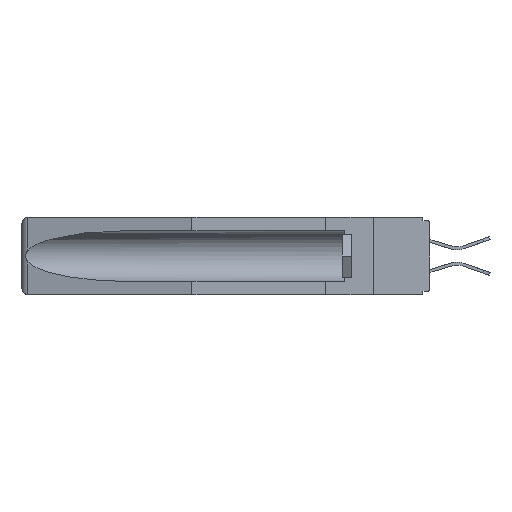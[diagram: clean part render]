
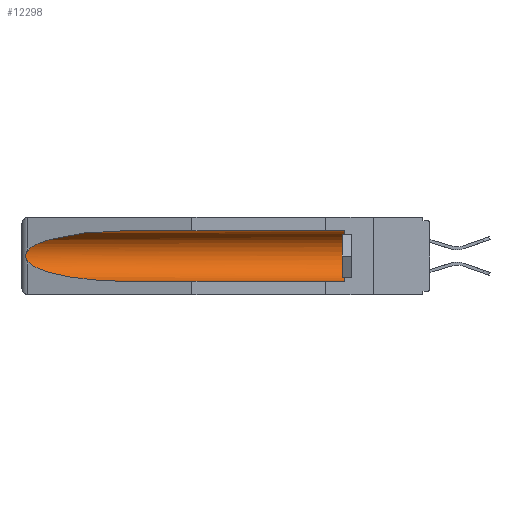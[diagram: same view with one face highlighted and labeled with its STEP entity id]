
A CAD part, left-side view. The second image highlights one B-rep face of the part: STEP entity #12298.
In plain terms, the highlighted cylindrical face has radius 2.857 mm (diameter 5.715 mm), a partial arc.
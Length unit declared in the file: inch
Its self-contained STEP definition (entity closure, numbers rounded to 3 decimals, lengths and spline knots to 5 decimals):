
#168 = CARTESIAN_POINT ( 'NONE',  ( 0.26597, 1.5296, -0.19026 ) ) ;
#405 = CARTESIAN_POINT ( 'NONE',  ( 0.2673, 1.53269, -0.17917 ) ) ;
#1002 = CARTESIAN_POINT ( 'NONE',  ( 0.155, 1.07973, -0.059 ) ) ;
#1911 = ORIENTED_EDGE ( 'NONE', *, *, #16237, .T. ) ;
#3357 = B_SPLINE_CURVE_WITH_KNOTS ( 'NONE', 3,
 ( #9916, #6105, #11764, #21163, #11851, #11530, #405, #13508, #168, #13671 ),
 .UNSPECIFIED., .F., .F.,
 ( 4, 2, 2, 2, 4 ),
 ( 0., 0.00029, 0.00058, 0.00087, 0.00117 ),
 .UNSPECIFIED. ) ;
#3642 = DIRECTION ( 'NONE',  ( 0., 0., 1. ) ) ;
#3734 = ORIENTED_EDGE ( 'NONE', *, *, #9068, .F. ) ;
#3971 = VECTOR ( 'NONE', #6389, 39.37008 ) ;
#4084 = AXIS2_PLACEMENT_3D ( 'NONE', #11189, #5364, #3642 ) ;
#4534 = CARTESIAN_POINT ( 'NONE',  ( 0.26537, 1.52718, -0.19328 ) ) ;
#5364 = DIRECTION ( 'NONE',  ( 0., 1., 0. ) ) ;
#5437 = DIRECTION ( 'NONE',  ( 0., 0., 1. ) ) ;
#5615 = CARTESIAN_POINT ( 'NONE',  ( 0.155, 0.126, -0.1715 ) ) ;
#6105 = CARTESIAN_POINT ( 'NONE',  ( 0.26597, 1.52961, -0.15275 ) ) ;
#6367 = EDGE_CURVE ( 'NONE', #6925, #9127, #13152, .T. ) ;
#6389 = DIRECTION ( 'NONE',  ( 0., 1., 0. ) ) ;
#6392 = CARTESIAN_POINT ( 'NONE',  ( 0.21114, 1.30732, -0.284 ) ) ;
#6740 = CYLINDRICAL_SURFACE ( 'NONE', #4084, 0.1125 ) ;
#6925 = VERTEX_POINT ( 'NONE', #13008 ) ;
#7333 = CARTESIAN_POINT ( 'NONE',  ( 0.155, -0.30754, -0.059 ) ) ;
#7741 = AXIS2_PLACEMENT_3D ( 'NONE', #5615, #9327, #5437 ) ;
#7800 = EDGE_CURVE ( 'NONE', #15560, #8006, #3357, .T. ) ;
#8006 = VERTEX_POINT ( 'NONE', #4534 ) ;
#8817 = FACE_OUTER_BOUND ( 'NONE', #18758, .T. ) ;
#9068 = EDGE_CURVE ( 'NONE', #17159, #22945, #17470, .T. ) ;
#9127 = VERTEX_POINT ( 'NONE', #13277 ) ;
#9134 = ORIENTED_EDGE ( 'NONE', *, *, #6367, .T. ) ;
#9327 = DIRECTION ( 'NONE',  ( 0., -1., 0. ) ) ;
#9916 = CARTESIAN_POINT ( 'NONE',  ( 0.26537, 1.52718, -0.14972 ) ) ;
#10956 = DIRECTION ( 'NONE',  ( 0., 1., 0. ) ) ;
#11189 = CARTESIAN_POINT ( 'NONE',  ( 0.155, -0.30754, -0.1715 ) ) ;
#11530 = CARTESIAN_POINT ( 'NONE',  ( 0.2675, 1.53308, -0.17534 ) ) ;
#11764 = CARTESIAN_POINT ( 'NONE',  ( 0.26654, 1.53092, -0.15636 ) ) ;
#11851 = CARTESIAN_POINT ( 'NONE',  ( 0.2675, 1.53308, -0.16763 ) ) ;
#12298 = ADVANCED_FACE ( 'NONE', ( #8817 ), #6740, .F. ) ;
#13008 = CARTESIAN_POINT ( 'NONE',  ( 0.155, 0.126, -0.059 ) ) ;
#13152 = LINE ( 'NONE', #7333, #3971 ) ;
#13276 = ORIENTED_EDGE ( 'NONE', *, *, #7800, .T. ) ;
#13277 = CARTESIAN_POINT ( 'NONE',  ( 0.155, 1.07973, -0.059 ) ) ;
#13508 = CARTESIAN_POINT ( 'NONE',  ( 0.26655, 1.53094, -0.18657 ) ) ;
#13671 = CARTESIAN_POINT ( 'NONE',  ( 0.26537, 1.52718, -0.19328 ) ) ;
#14154 = EDGE_CURVE ( 'NONE', #9127, #15560, #22742, .T. ) ;
#14417 = CARTESIAN_POINT ( 'NONE',  ( 0.26537, 1.52718, -0.14972 ) ) ;
#14963 = CARTESIAN_POINT ( 'NONE',  ( 0.155, 0.126, -0.284 ) ) ;
#15560 = VERTEX_POINT ( 'NONE', #19861 ) ;
#16156 = CARTESIAN_POINT ( 'NONE',  ( 0.21114, 1.30732, -0.059 ) ) ;
#16237 = EDGE_CURVE ( 'NONE', #8006, #22945, #20940, .T. ) ;
#16647 = CARTESIAN_POINT ( 'NONE',  ( 0.155, -0.30754, -0.284 ) ) ;
#17159 = VERTEX_POINT ( 'NONE', #14963 ) ;
#17470 = LINE ( 'NONE', #16647, #17757 ) ;
#17757 = VECTOR ( 'NONE', #10956, 39.37008 ) ;
#18758 = EDGE_LOOP ( 'NONE', ( #23202, #13276, #1911, #3734, #22509, #9134 ) ) ;
#19003 = CARTESIAN_POINT ( 'NONE',  ( 0.155, 1.07973, -0.284 ) ) ;
#19468 = CARTESIAN_POINT ( 'NONE',  ( 0.25451, 1.48313, -0.24835 ) ) ;
#19539 = CARTESIAN_POINT ( 'NONE',  ( 0.26537, 1.52718, -0.19328 ) ) ;
#19668 = CIRCLE ( 'NONE', #7741, 0.1125 ) ;
#19699 = CARTESIAN_POINT ( 'NONE',  ( 0.155, 1.07973, -0.284 ) ) ;
#19861 = CARTESIAN_POINT ( 'NONE',  ( 0.26537, 1.52718, -0.14972 ) ) ;
#20940 =( BOUNDED_CURVE ( )  B_SPLINE_CURVE ( 3, ( #19539, #19468, #6392, #19699 ),
 .UNSPECIFIED., .F., .F. ) 
 B_SPLINE_CURVE_WITH_KNOTS ( ( 4, 4 ),
 ( 0.1948, 1.5708 ),
 .UNSPECIFIED. ) 
 CURVE ( )  GEOMETRIC_REPRESENTATION_ITEM ( )  RATIONAL_B_SPLINE_CURVE ( ( 1., 0.848, 0.848, 1. ) ) 
 REPRESENTATION_ITEM ( '' )  );
#21163 = CARTESIAN_POINT ( 'NONE',  ( 0.2673, 1.5327, -0.16383 ) ) ;
#21982 = CARTESIAN_POINT ( 'NONE',  ( 0.25451, 1.48313, -0.09465 ) ) ;
#22072 = EDGE_CURVE ( 'NONE', #17159, #6925, #19668, .T. ) ;
#22509 = ORIENTED_EDGE ( 'NONE', *, *, #22072, .T. ) ;
#22742 =( BOUNDED_CURVE ( )  B_SPLINE_CURVE ( 3, ( #1002, #16156, #21982, #14417 ),
 .UNSPECIFIED., .F., .F. ) 
 B_SPLINE_CURVE_WITH_KNOTS ( ( 4, 4 ),
 ( 4.71239, 6.08839 ),
 .UNSPECIFIED. ) 
 CURVE ( )  GEOMETRIC_REPRESENTATION_ITEM ( )  RATIONAL_B_SPLINE_CURVE ( ( 1., 0.848, 0.848, 1. ) ) 
 REPRESENTATION_ITEM ( '' )  );
#22945 = VERTEX_POINT ( 'NONE', #19003 ) ;
#23202 = ORIENTED_EDGE ( 'NONE', *, *, #14154, .T. ) ;
